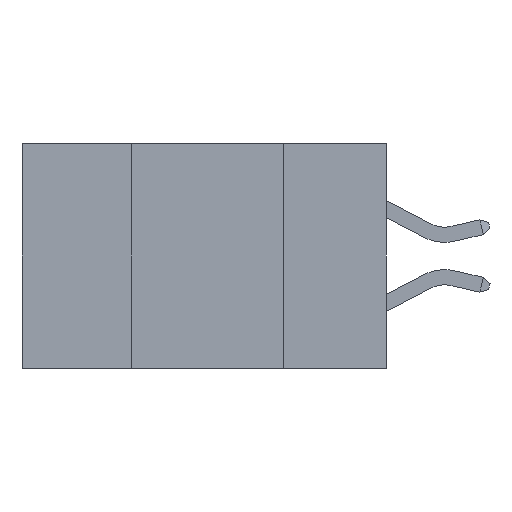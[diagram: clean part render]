
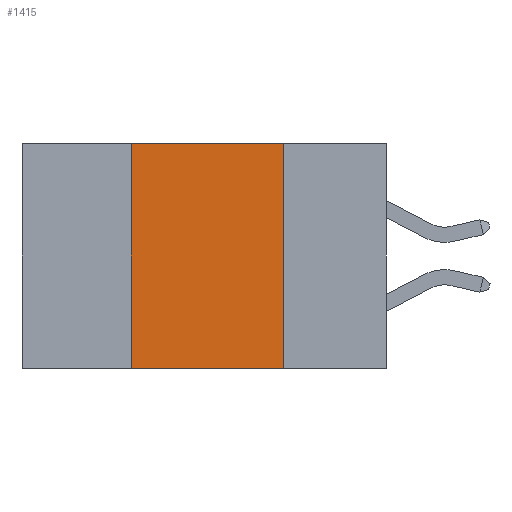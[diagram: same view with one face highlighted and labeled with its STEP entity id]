
A CAD part, left-side view. The second image highlights one B-rep face of the part: STEP entity #1415.
In plain terms, the highlighted planar face has unit normal (-1, 0, 0).
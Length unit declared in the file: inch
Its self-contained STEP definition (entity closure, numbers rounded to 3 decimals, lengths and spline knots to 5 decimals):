
#383 = VERTEX_POINT ( 'NONE', #3429 ) ;
#421 = EDGE_LOOP ( 'NONE', ( #5492, #14341, #16355, #593 ) ) ;
#593 = ORIENTED_EDGE ( 'NONE', *, *, #18335, .T. ) ;
#650 = EDGE_CURVE ( 'NONE', #2300, #3663, #13078, .T. ) ;
#748 = PLANE ( 'NONE',  #16496 ) ;
#1415 = ADVANCED_FACE ( 'NONE', ( #16171 ), #748, .F. ) ;
#1685 = EDGE_CURVE ( 'NONE', #383, #15664, #5527, .T. ) ;
#2300 = VERTEX_POINT ( 'NONE', #11602 ) ;
#2670 = EDGE_CURVE ( 'NONE', #3663, #383, #9055, .T. ) ;
#3429 = CARTESIAN_POINT ( 'NONE',  ( 0., 0.17, 0. ) ) ;
#3663 = VERTEX_POINT ( 'NONE', #14270 ) ;
#3847 = DIRECTION ( 'NONE',  ( 1., 0., 0. ) ) ;
#4051 = DIRECTION ( 'NONE',  ( 0., 0., 1. ) ) ;
#4142 = VECTOR ( 'NONE', #8654, 39.37008 ) ;
#5492 = ORIENTED_EDGE ( 'NONE', *, *, #1685, .F. ) ;
#5527 = LINE ( 'NONE', #15789, #12168 ) ;
#5688 = DIRECTION ( 'NONE',  ( 0., 0., -1. ) ) ;
#8529 = CARTESIAN_POINT ( 'NONE',  ( 0., 0.17, -0.37 ) ) ;
#8654 = DIRECTION ( 'NONE',  ( 0., -1., 0. ) ) ;
#9055 = LINE ( 'NONE', #15361, #16109 ) ;
#11356 = CARTESIAN_POINT ( 'NONE',  ( 0., 0.42, -0.37 ) ) ;
#11602 = CARTESIAN_POINT ( 'NONE',  ( 0., 0.42, -0.37 ) ) ;
#11732 = LINE ( 'NONE', #14232, #4142 ) ;
#12168 = VECTOR ( 'NONE', #5688, 39.37008 ) ;
#12631 = VECTOR ( 'NONE', #4051, 39.37008 ) ;
#13078 = LINE ( 'NONE', #11356, #12631 ) ;
#14232 = CARTESIAN_POINT ( 'NONE',  ( 0., 0.6, -0.37 ) ) ;
#14270 = CARTESIAN_POINT ( 'NONE',  ( 0., 0.42, 0. ) ) ;
#14341 = ORIENTED_EDGE ( 'NONE', *, *, #2670, .F. ) ;
#14597 = CARTESIAN_POINT ( 'NONE',  ( 0., 0.6, 0. ) ) ;
#15068 = DIRECTION ( 'NONE',  ( 0., 0., -1. ) ) ;
#15280 = DIRECTION ( 'NONE',  ( 0., -1., 0. ) ) ;
#15361 = CARTESIAN_POINT ( 'NONE',  ( 0., 0.6, 0. ) ) ;
#15664 = VERTEX_POINT ( 'NONE', #8529 ) ;
#15789 = CARTESIAN_POINT ( 'NONE',  ( 0., 0.17, -0.37 ) ) ;
#16109 = VECTOR ( 'NONE', #15280, 39.37008 ) ;
#16171 = FACE_OUTER_BOUND ( 'NONE', #421, .T. ) ;
#16355 = ORIENTED_EDGE ( 'NONE', *, *, #650, .F. ) ;
#16496 = AXIS2_PLACEMENT_3D ( 'NONE', #14597, #3847, #15068 ) ;
#18335 = EDGE_CURVE ( 'NONE', #2300, #15664, #11732, .T. ) ;
